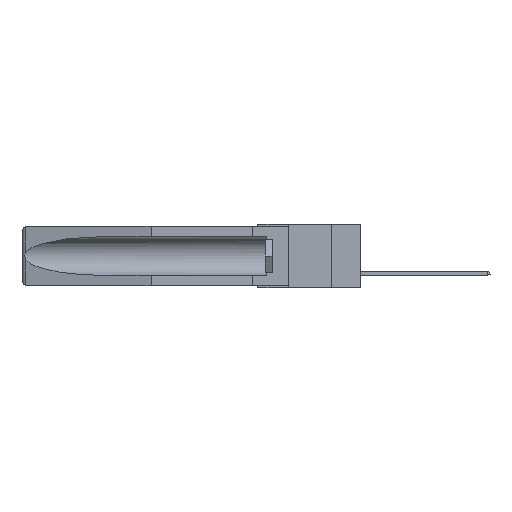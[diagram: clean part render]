
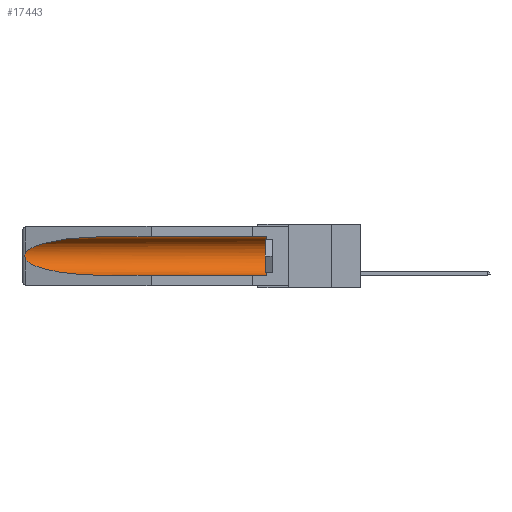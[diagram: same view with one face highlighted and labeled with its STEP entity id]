
A CAD part, left-side view. The second image highlights one B-rep face of the part: STEP entity #17443.
In plain terms, the highlighted cylindrical face has radius 2.857 mm (diameter 5.715 mm), a partial arc.
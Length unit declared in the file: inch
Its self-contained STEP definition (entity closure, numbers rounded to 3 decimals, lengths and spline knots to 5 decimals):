
#1011 = CARTESIAN_POINT ( 'NONE',  ( 0.26655, 1.53094, -0.18657 ) ) ;
#1224 = CIRCLE ( 'NONE', #8040, 0.1125 ) ;
#1504 = LINE ( 'NONE', #23537, #19592 ) ;
#1753 = DIRECTION ( 'NONE',  ( 0., 0., 1. ) ) ;
#1836 = VERTEX_POINT ( 'NONE', #27226 ) ;
#2981 = VERTEX_POINT ( 'NONE', #18635 ) ;
#3723 = EDGE_CURVE ( 'NONE', #1836, #23866, #32582, .T. ) ;
#4476 = CARTESIAN_POINT ( 'NONE',  ( 0.26537, 1.52718, -0.14972 ) ) ;
#5319 = CARTESIAN_POINT ( 'NONE',  ( 0.155, 1.07973, -0.059 ) ) ;
#6079 = CARTESIAN_POINT ( 'NONE',  ( 0.26597, 1.52961, -0.15275 ) ) ;
#6351 = VERTEX_POINT ( 'NONE', #7666 ) ;
#6419 = DIRECTION ( 'NONE',  ( 0., 1., 0. ) ) ;
#6768 = ORIENTED_EDGE ( 'NONE', *, *, #3723, .T. ) ;
#7115 = CARTESIAN_POINT ( 'NONE',  ( 0.155, 1.07973, -0.284 ) ) ;
#7246 = EDGE_CURVE ( 'NONE', #15568, #1836, #10578, .T. ) ;
#7666 = CARTESIAN_POINT ( 'NONE',  ( 0.155, 0.126, -0.284 ) ) ;
#8040 = AXIS2_PLACEMENT_3D ( 'NONE', #14527, #19559, #1753 ) ;
#8367 = CARTESIAN_POINT ( 'NONE',  ( 0.2673, 1.5327, -0.16383 ) ) ;
#8487 = CARTESIAN_POINT ( 'NONE',  ( 0.26654, 1.53092, -0.15636 ) ) ;
#8612 = CARTESIAN_POINT ( 'NONE',  ( 0.21114, 1.30732, -0.284 ) ) ;
#9675 = ORIENTED_EDGE ( 'NONE', *, *, #29637, .T. ) ;
#9839 = CARTESIAN_POINT ( 'NONE',  ( 0.25451, 1.48313, -0.09465 ) ) ;
#10315 = FACE_OUTER_BOUND ( 'NONE', #28900, .T. ) ;
#10578 = B_SPLINE_CURVE_WITH_KNOTS ( 'NONE', 3,
 ( #11190, #6079, #8487, #8367, #10978, #31145, #11311, #1011, #13749, #10887 ),
 .UNSPECIFIED., .F., .F.,
 ( 4, 2, 2, 2, 4 ),
 ( 0., 0.00029, 0.00058, 0.00087, 0.00117 ),
 .UNSPECIFIED. ) ;
#10887 = CARTESIAN_POINT ( 'NONE',  ( 0.26537, 1.52718, -0.19328 ) ) ;
#10978 = CARTESIAN_POINT ( 'NONE',  ( 0.2675, 1.53308, -0.16763 ) ) ;
#11185 = EDGE_CURVE ( 'NONE', #6351, #23866, #1504, .T. ) ;
#11190 = CARTESIAN_POINT ( 'NONE',  ( 0.26537, 1.52718, -0.14972 ) ) ;
#11311 = CARTESIAN_POINT ( 'NONE',  ( 0.2673, 1.53269, -0.17917 ) ) ;
#11531 = DIRECTION ( 'NONE',  ( 0., 0., 1. ) ) ;
#13316 = ORIENTED_EDGE ( 'NONE', *, *, #7246, .T. ) ;
#13323 = CARTESIAN_POINT ( 'NONE',  ( 0.155, 1.07973, -0.059 ) ) ;
#13749 = CARTESIAN_POINT ( 'NONE',  ( 0.26597, 1.5296, -0.19026 ) ) ;
#14527 = CARTESIAN_POINT ( 'NONE',  ( 0.155, 0.126, -0.1715 ) ) ;
#15115 = CARTESIAN_POINT ( 'NONE',  ( 0.21114, 1.30732, -0.059 ) ) ;
#15568 = VERTEX_POINT ( 'NONE', #4476 ) ;
#16815 = CARTESIAN_POINT ( 'NONE',  ( 0.155, -0.30754, -0.059 ) ) ;
#17443 = ADVANCED_FACE ( 'NONE', ( #10315 ), #17779, .F. ) ;
#17628 = CARTESIAN_POINT ( 'NONE',  ( 0.26537, 1.52718, -0.14972 ) ) ;
#17779 = CYLINDRICAL_SURFACE ( 'NONE', #26307, 0.1125 ) ;
#17870 = ORIENTED_EDGE ( 'NONE', *, *, #22443, .T. ) ;
#18230 =( BOUNDED_CURVE ( )  B_SPLINE_CURVE ( 3, ( #5319, #15115, #9839, #17628 ),
 .UNSPECIFIED., .F., .T. ) 
 B_SPLINE_CURVE_WITH_KNOTS ( ( 4, 4 ),
 ( 4.71239, 6.08839 ),
 .UNSPECIFIED. ) 
 CURVE ( )  GEOMETRIC_REPRESENTATION_ITEM ( )  RATIONAL_B_SPLINE_CURVE ( ( 1., 0.848, 0.848, 1. ) ) 
 REPRESENTATION_ITEM ( '' )  );
#18577 = CARTESIAN_POINT ( 'NONE',  ( 0.26537, 1.52718, -0.19328 ) ) ;
#18635 = CARTESIAN_POINT ( 'NONE',  ( 0.155, 0.126, -0.059 ) ) ;
#19559 = DIRECTION ( 'NONE',  ( 0., -1., 0. ) ) ;
#19592 = VECTOR ( 'NONE', #25977, 39.37008 ) ;
#20872 = EDGE_CURVE ( 'NONE', #2981, #22371, #31053, .T. ) ;
#20924 = ORIENTED_EDGE ( 'NONE', *, *, #11185, .F. ) ;
#21471 = CARTESIAN_POINT ( 'NONE',  ( 0.155, -0.30754, -0.1715 ) ) ;
#21985 = DIRECTION ( 'NONE',  ( 0., 1., 0. ) ) ;
#22371 = VERTEX_POINT ( 'NONE', #13323 ) ;
#22443 = EDGE_CURVE ( 'NONE', #6351, #2981, #1224, .T. ) ;
#23537 = CARTESIAN_POINT ( 'NONE',  ( 0.155, -0.30754, -0.284 ) ) ;
#23866 = VERTEX_POINT ( 'NONE', #7115 ) ;
#25067 = ORIENTED_EDGE ( 'NONE', *, *, #20872, .T. ) ;
#25977 = DIRECTION ( 'NONE',  ( 0., 1., 0. ) ) ;
#26307 = AXIS2_PLACEMENT_3D ( 'NONE', #21471, #6419, #11531 ) ;
#27226 = CARTESIAN_POINT ( 'NONE',  ( 0.26537, 1.52718, -0.19328 ) ) ;
#28754 = CARTESIAN_POINT ( 'NONE',  ( 0.25451, 1.48313, -0.24835 ) ) ;
#28900 = EDGE_LOOP ( 'NONE', ( #9675, #13316, #6768, #20924, #17870, #25067 ) ) ;
#28972 = CARTESIAN_POINT ( 'NONE',  ( 0.155, 1.07973, -0.284 ) ) ;
#29637 = EDGE_CURVE ( 'NONE', #22371, #15568, #18230, .T. ) ;
#31053 = LINE ( 'NONE', #16815, #32251 ) ;
#31145 = CARTESIAN_POINT ( 'NONE',  ( 0.2675, 1.53308, -0.17534 ) ) ;
#32251 = VECTOR ( 'NONE', #21985, 39.37008 ) ;
#32582 =( BOUNDED_CURVE ( )  B_SPLINE_CURVE ( 3, ( #18577, #28754, #8612, #28972 ),
 .UNSPECIFIED., .F., .F. ) 
 B_SPLINE_CURVE_WITH_KNOTS ( ( 4, 4 ),
 ( 0.1948, 1.5708 ),
 .UNSPECIFIED. ) 
 CURVE ( )  GEOMETRIC_REPRESENTATION_ITEM ( )  RATIONAL_B_SPLINE_CURVE ( ( 1., 0.848, 0.848, 1. ) ) 
 REPRESENTATION_ITEM ( '' )  );
